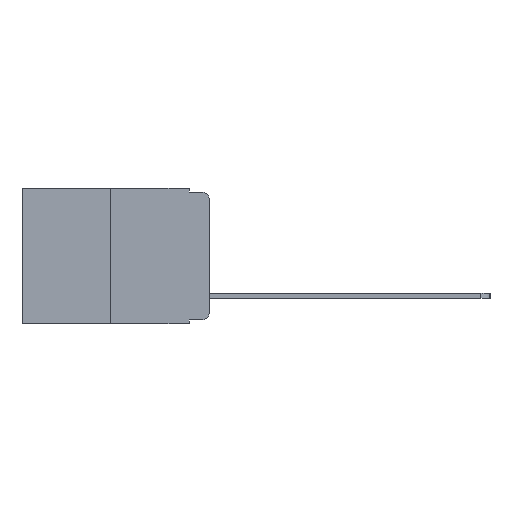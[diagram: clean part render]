
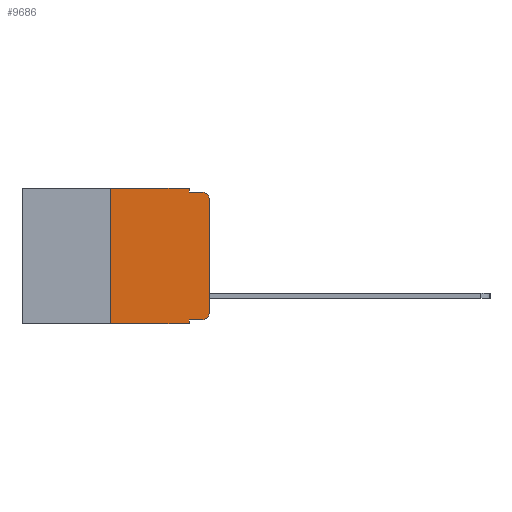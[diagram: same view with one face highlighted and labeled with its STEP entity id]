
A CAD part, left-side view. The second image highlights one B-rep face of the part: STEP entity #9686.
In plain terms, the highlighted planar face has unit normal (-1, 0, 0).
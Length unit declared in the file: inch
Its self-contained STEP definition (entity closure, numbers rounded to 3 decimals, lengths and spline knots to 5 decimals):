
#139 = LINE ( 'NONE', #1278, #3312 ) ;
#1278 = CARTESIAN_POINT ( 'NONE',  ( 0., 0.051, 0. ) ) ;
#1353 = DIRECTION ( 'NONE',  ( 0., 0., -1. ) ) ;
#2119 = VECTOR ( 'NONE', #8876, 39.37008 ) ;
#2233 = EDGE_LOOP ( 'NONE', ( #7285, #12538, #21744, #3544, #18239, #22815, #5312, #10013, #11152, #15813 ) ) ;
#2867 = AXIS2_PLACEMENT_3D ( 'NONE', #9097, #21310, #10873 ) ;
#3312 = VECTOR ( 'NONE', #6839, 39.37008 ) ;
#3396 = VECTOR ( 'NONE', #14277, 39.37008 ) ;
#3499 = CARTESIAN_POINT ( 'NONE',  ( 0., 0.473, 0. ) ) ;
#3544 = ORIENTED_EDGE ( 'NONE', *, *, #9684, .F. ) ;
#3552 = LINE ( 'NONE', #10232, #21751 ) ;
#3571 = CARTESIAN_POINT ( 'NONE',  ( 0., 0.051, 0. ) ) ;
#3921 = CIRCLE ( 'NONE', #15475, 0.02 ) ;
#4259 = CARTESIAN_POINT ( 'NONE',  ( 0., 0.051, -0.333 ) ) ;
#4687 = VERTEX_POINT ( 'NONE', #6711 ) ;
#5265 = LINE ( 'NONE', #7719, #13582 ) ;
#5312 = ORIENTED_EDGE ( 'NONE', *, *, #11965, .T. ) ;
#5609 = DIRECTION ( 'NONE',  ( 0., -1., 0. ) ) ;
#5848 = VERTEX_POINT ( 'NONE', #20787 ) ;
#6159 = EDGE_CURVE ( 'NONE', #5848, #12563, #5265, .T. ) ;
#6378 = DIRECTION ( 'NONE',  ( 0., -1., 0. ) ) ;
#6711 = CARTESIAN_POINT ( 'NONE',  ( 0., 0.02, -0.01 ) ) ;
#6822 = VERTEX_POINT ( 'NONE', #15145 ) ;
#6839 = DIRECTION ( 'NONE',  ( 0., 0., -1. ) ) ;
#7285 = ORIENTED_EDGE ( 'NONE', *, *, #14019, .T. ) ;
#7719 = CARTESIAN_POINT ( 'NONE',  ( 0., 0.25, 0. ) ) ;
#8106 = EDGE_CURVE ( 'NONE', #8656, #4687, #9588, .T. ) ;
#8656 = VERTEX_POINT ( 'NONE', #10411 ) ;
#8876 = DIRECTION ( 'NONE',  ( 0., -1., 0. ) ) ;
#9083 = CARTESIAN_POINT ( 'NONE',  ( 0., 0.02, -0.03 ) ) ;
#9094 = CARTESIAN_POINT ( 'NONE',  ( 0., 0.473, -0.343 ) ) ;
#9097 = CARTESIAN_POINT ( 'NONE',  ( 0., 0.02, -0.313 ) ) ;
#9265 = EDGE_CURVE ( 'NONE', #10346, #4687, #3921, .T. ) ;
#9588 = LINE ( 'NONE', #22099, #22946 ) ;
#9684 = EDGE_CURVE ( 'NONE', #6822, #8656, #139, .T. ) ;
#9686 = ADVANCED_FACE ( 'NONE', ( #16957 ), #17356, .F. ) ;
#9881 = LINE ( 'NONE', #11087, #18659 ) ;
#10013 = ORIENTED_EDGE ( 'NONE', *, *, #19526, .F. ) ;
#10232 = CARTESIAN_POINT ( 'NONE',  ( 0., 0., 0. ) ) ;
#10346 = VERTEX_POINT ( 'NONE', #20500 ) ;
#10411 = CARTESIAN_POINT ( 'NONE',  ( 0., 0.051, -0.01 ) ) ;
#10608 = EDGE_CURVE ( 'NONE', #12563, #6822, #20961, .T. ) ;
#10852 = DIRECTION ( 'NONE',  ( 0., 0., -1. ) ) ;
#10873 = DIRECTION ( 'NONE',  ( 0., 0., -1. ) ) ;
#11087 = CARTESIAN_POINT ( 'NONE',  ( 0., 0.051, -0.333 ) ) ;
#11152 = ORIENTED_EDGE ( 'NONE', *, *, #18357, .T. ) ;
#11965 = EDGE_CURVE ( 'NONE', #5848, #14326, #20252, .T. ) ;
#12182 = DIRECTION ( 'NONE',  ( 1., 0., 0. ) ) ;
#12538 = ORIENTED_EDGE ( 'NONE', *, *, #9265, .T. ) ;
#12563 = VERTEX_POINT ( 'NONE', #21278 ) ;
#12580 = VERTEX_POINT ( 'NONE', #19548 ) ;
#13103 = CARTESIAN_POINT ( 'NONE',  ( 0., 0.051, -0.343 ) ) ;
#13582 = VECTOR ( 'NONE', #18189, 39.37008 ) ;
#13803 = DIRECTION ( 'NONE',  ( 0., 0., 1. ) ) ;
#14019 = EDGE_CURVE ( 'NONE', #22000, #10346, #3552, .T. ) ;
#14277 = DIRECTION ( 'NONE',  ( 0., 0., -1. ) ) ;
#14326 = VERTEX_POINT ( 'NONE', #13103 ) ;
#15145 = CARTESIAN_POINT ( 'NONE',  ( 0., 0.051, 0. ) ) ;
#15475 = AXIS2_PLACEMENT_3D ( 'NONE', #9083, #21290, #10852 ) ;
#15776 = AXIS2_PLACEMENT_3D ( 'NONE', #22541, #12182, #1353 ) ;
#15813 = ORIENTED_EDGE ( 'NONE', *, *, #16041, .T. ) ;
#16041 = EDGE_CURVE ( 'NONE', #12580, #22000, #22352, .T. ) ;
#16957 = FACE_OUTER_BOUND ( 'NONE', #2233, .T. ) ;
#17356 = PLANE ( 'NONE',  #15776 ) ;
#18118 = DIRECTION ( 'NONE',  ( 0., -1., 0. ) ) ;
#18189 = DIRECTION ( 'NONE',  ( 0., 0., 1. ) ) ;
#18239 = ORIENTED_EDGE ( 'NONE', *, *, #10608, .F. ) ;
#18357 = EDGE_CURVE ( 'NONE', #22831, #12580, #9881, .T. ) ;
#18659 = VECTOR ( 'NONE', #18118, 39.37008 ) ;
#19160 = VECTOR ( 'NONE', #5609, 39.37008 ) ;
#19526 = EDGE_CURVE ( 'NONE', #22831, #14326, #22679, .T. ) ;
#19548 = CARTESIAN_POINT ( 'NONE',  ( 0., 0.02, -0.333 ) ) ;
#20252 = LINE ( 'NONE', #9094, #19160 ) ;
#20373 = CARTESIAN_POINT ( 'NONE',  ( 0., 0., -0.313 ) ) ;
#20500 = CARTESIAN_POINT ( 'NONE',  ( 0., 0., -0.03 ) ) ;
#20787 = CARTESIAN_POINT ( 'NONE',  ( 0., 0.25, -0.343 ) ) ;
#20961 = LINE ( 'NONE', #3499, #2119 ) ;
#21278 = CARTESIAN_POINT ( 'NONE',  ( 0., 0.25, 0. ) ) ;
#21290 = DIRECTION ( 'NONE',  ( -1., 0., 0. ) ) ;
#21310 = DIRECTION ( 'NONE',  ( -1., 0., 0. ) ) ;
#21744 = ORIENTED_EDGE ( 'NONE', *, *, #8106, .F. ) ;
#21751 = VECTOR ( 'NONE', #13803, 39.37008 ) ;
#22000 = VERTEX_POINT ( 'NONE', #20373 ) ;
#22099 = CARTESIAN_POINT ( 'NONE',  ( 0., 0.051, -0.01 ) ) ;
#22352 = CIRCLE ( 'NONE', #2867, 0.02 ) ;
#22541 = CARTESIAN_POINT ( 'NONE',  ( 0., 0.473, 0. ) ) ;
#22679 = LINE ( 'NONE', #3571, #3396 ) ;
#22815 = ORIENTED_EDGE ( 'NONE', *, *, #6159, .F. ) ;
#22831 = VERTEX_POINT ( 'NONE', #4259 ) ;
#22946 = VECTOR ( 'NONE', #6378, 39.37008 ) ;
